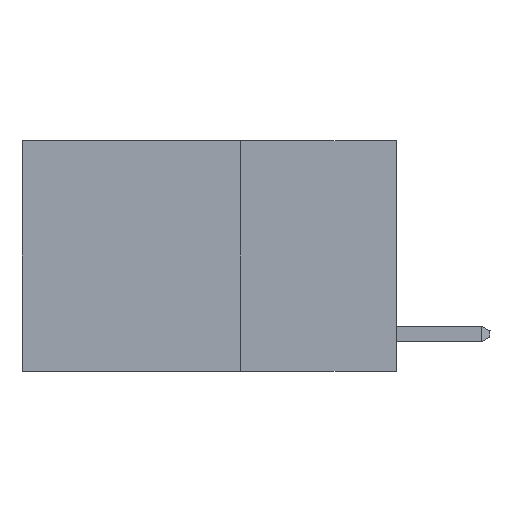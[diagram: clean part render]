
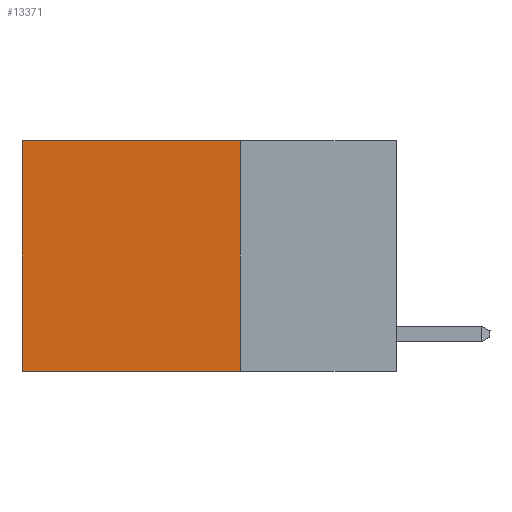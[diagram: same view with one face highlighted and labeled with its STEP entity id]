
A CAD part, left-side view. The second image highlights one B-rep face of the part: STEP entity #13371.
In plain terms, the highlighted planar face has unit normal (-1, 0, 0).
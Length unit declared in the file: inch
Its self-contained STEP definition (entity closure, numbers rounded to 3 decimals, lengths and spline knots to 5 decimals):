
#1146 = VERTEX_POINT ( 'NONE', #14629 ) ;
#1165 = ORIENTED_EDGE ( 'NONE', *, *, #4296, .F. ) ;
#1603 = DIRECTION ( 'NONE',  ( 1., 0., 0. ) ) ;
#1831 = EDGE_CURVE ( 'NONE', #12649, #12934, #5135, .T. ) ;
#2735 = VERTEX_POINT ( 'NONE', #15365 ) ;
#3040 = ORIENTED_EDGE ( 'NONE', *, *, #1831, .T. ) ;
#3498 = PLANE ( 'NONE',  #8815 ) ;
#3562 = VECTOR ( 'NONE', #19461, 39.37008 ) ;
#4296 = EDGE_CURVE ( 'NONE', #1146, #12934, #11563, .T. ) ;
#5135 = LINE ( 'NONE', #20996, #3562 ) ;
#6756 = EDGE_CURVE ( 'NONE', #2735, #12649, #13916, .T. ) ;
#6939 = CARTESIAN_POINT ( 'NONE',  ( 0.2625, 0.6, -0.37 ) ) ;
#7267 = ORIENTED_EDGE ( 'NONE', *, *, #14575, .F. ) ;
#7583 = VECTOR ( 'NONE', #21814, 39.37008 ) ;
#8382 = CARTESIAN_POINT ( 'NONE',  ( 0.2625, 0.25, 0. ) ) ;
#8455 = DIRECTION ( 'NONE',  ( 0., 0., -1. ) ) ;
#8815 = AXIS2_PLACEMENT_3D ( 'NONE', #8382, #1603, #8455 ) ;
#10695 = CARTESIAN_POINT ( 'NONE',  ( 0.2625, 0.6, 0. ) ) ;
#11404 = DIRECTION ( 'NONE',  ( 0., 1., 0. ) ) ;
#11563 = LINE ( 'NONE', #11735, #7583 ) ;
#11735 = CARTESIAN_POINT ( 'NONE',  ( 0.2625, 0.25, -0.37 ) ) ;
#12649 = VERTEX_POINT ( 'NONE', #10695 ) ;
#12934 = VERTEX_POINT ( 'NONE', #6939 ) ;
#13371 = ADVANCED_FACE ( 'NONE', ( #18310 ), #3498, .F. ) ;
#13730 = LINE ( 'NONE', #17186, #18713 ) ;
#13833 = EDGE_LOOP ( 'NONE', ( #3040, #1165, #7267, #15411 ) ) ;
#13916 = LINE ( 'NONE', #15190, #19450 ) ;
#14467 = DIRECTION ( 'NONE',  ( 0., 0., -1. ) ) ;
#14575 = EDGE_CURVE ( 'NONE', #2735, #1146, #13730, .T. ) ;
#14629 = CARTESIAN_POINT ( 'NONE',  ( 0.2625, 0.25, -0.37 ) ) ;
#15190 = CARTESIAN_POINT ( 'NONE',  ( 0.2625, 0.25, 0. ) ) ;
#15365 = CARTESIAN_POINT ( 'NONE',  ( 0.2625, 0.25, 0. ) ) ;
#15411 = ORIENTED_EDGE ( 'NONE', *, *, #6756, .T. ) ;
#17186 = CARTESIAN_POINT ( 'NONE',  ( 0.2625, 0.25, 0. ) ) ;
#18310 = FACE_OUTER_BOUND ( 'NONE', #13833, .T. ) ;
#18713 = VECTOR ( 'NONE', #14467, 39.37008 ) ;
#19450 = VECTOR ( 'NONE', #11404, 39.37008 ) ;
#19461 = DIRECTION ( 'NONE',  ( 0., 0., -1. ) ) ;
#20996 = CARTESIAN_POINT ( 'NONE',  ( 0.2625, 0.6, 0. ) ) ;
#21814 = DIRECTION ( 'NONE',  ( 0., 1., 0. ) ) ;
